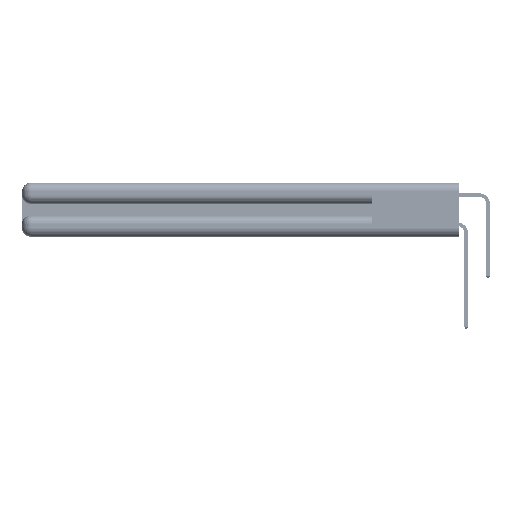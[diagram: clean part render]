
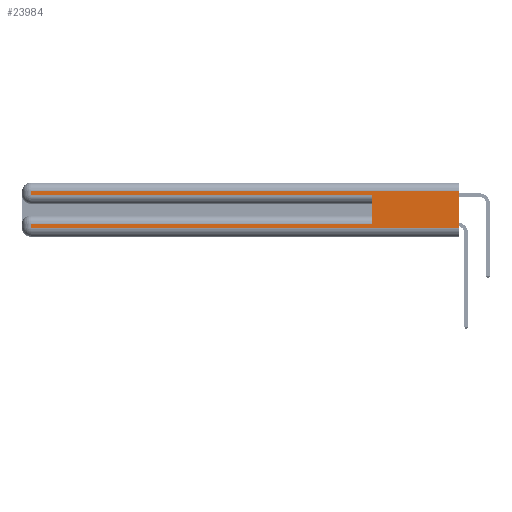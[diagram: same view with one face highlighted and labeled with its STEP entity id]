
A CAD part, left-side view. The second image highlights one B-rep face of the part: STEP entity #23984.
In plain terms, the highlighted planar face has unit normal (-1, 0, 0).
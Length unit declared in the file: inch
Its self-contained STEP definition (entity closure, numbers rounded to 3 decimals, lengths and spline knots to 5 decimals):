
#96 = FACE_OUTER_BOUND ( 'NONE', #7727, .T. ) ;
#660 = EDGE_CURVE ( 'NONE', #20867, #53211, #20556, .T. ) ;
#1240 = EDGE_CURVE ( 'NONE', #20867, #17692, #34169, .T. ) ;
#1460 = CARTESIAN_POINT ( 'NONE',  ( 0., 0., 0.06 ) ) ;
#1725 = LINE ( 'NONE', #55811, #45574 ) ;
#2793 = CARTESIAN_POINT ( 'NONE',  ( 0., 2.94, 0.37 ) ) ;
#4167 = VECTOR ( 'NONE', #28783, 39.37008 ) ;
#4797 = CARTESIAN_POINT ( 'NONE',  ( 0., 0., 0.31 ) ) ;
#5578 = CARTESIAN_POINT ( 'NONE',  ( 0., 0., 0.06 ) ) ;
#5601 = ORIENTED_EDGE ( 'NONE', *, *, #31787, .T. ) ;
#6433 = VECTOR ( 'NONE', #7778, 39.37008 ) ;
#7390 = CARTESIAN_POINT ( 'NONE',  ( 0., 0., 0.285 ) ) ;
#7727 = EDGE_LOOP ( 'NONE', ( #41674, #23294, #35686, #5601, #39688, #41686, #26981, #34441 ) ) ;
#7778 = DIRECTION ( 'NONE',  ( 0., -1., 0. ) ) ;
#8100 = DIRECTION ( 'NONE',  ( 1., 0., 0. ) ) ;
#8307 = LINE ( 'NONE', #28275, #26051 ) ;
#10941 = VECTOR ( 'NONE', #50600, 39.37008 ) ;
#12509 = VECTOR ( 'NONE', #22643, 39.37008 ) ;
#12558 = VERTEX_POINT ( 'NONE', #35543 ) ;
#12775 = VERTEX_POINT ( 'NONE', #15792 ) ;
#14449 = CARTESIAN_POINT ( 'NONE',  ( 0., 0., 0.085 ) ) ;
#15102 = VERTEX_POINT ( 'NONE', #45739 ) ;
#15792 = CARTESIAN_POINT ( 'NONE',  ( 0., 2.94, 0.285 ) ) ;
#17211 = VECTOR ( 'NONE', #40591, 39.37008 ) ;
#17470 = CARTESIAN_POINT ( 'NONE',  ( 0., 2.94, 0.31 ) ) ;
#17692 = VERTEX_POINT ( 'NONE', #1460 ) ;
#19238 = EDGE_CURVE ( 'NONE', #26409, #15102, #8307, .T. ) ;
#20556 = LINE ( 'NONE', #54392, #42480 ) ;
#20867 = VERTEX_POINT ( 'NONE', #4797 ) ;
#22643 = DIRECTION ( 'NONE',  ( 0., 1., 0. ) ) ;
#22738 = LINE ( 'NONE', #14449, #12509 ) ;
#23294 = ORIENTED_EDGE ( 'NONE', *, *, #660, .T. ) ;
#23572 = EDGE_CURVE ( 'NONE', #12558, #26409, #22738, .T. ) ;
#23984 = ADVANCED_FACE ( 'NONE', ( #96 ), #25264, .F. ) ;
#25075 = EDGE_CURVE ( 'NONE', #53211, #12775, #39094, .T. ) ;
#25264 = PLANE ( 'NONE',  #39997 ) ;
#26051 = VECTOR ( 'NONE', #43010, 39.37008 ) ;
#26409 = VERTEX_POINT ( 'NONE', #36772 ) ;
#26981 = ORIENTED_EDGE ( 'NONE', *, *, #19238, .T. ) ;
#28035 = EDGE_CURVE ( 'NONE', #12558, #34216, #1725, .T. ) ;
#28117 = DIRECTION ( 'NONE',  ( 0., 1., 0. ) ) ;
#28275 = CARTESIAN_POINT ( 'NONE',  ( 0., 2.94, 0.37 ) ) ;
#28783 = DIRECTION ( 'NONE',  ( 0., 0., -1. ) ) ;
#31787 = EDGE_CURVE ( 'NONE', #12775, #34216, #51623, .T. ) ;
#34169 = LINE ( 'NONE', #50782, #10941 ) ;
#34216 = VERTEX_POINT ( 'NONE', #39833 ) ;
#34277 = CARTESIAN_POINT ( 'NONE',  ( 0., 0., 0.37 ) ) ;
#34441 = ORIENTED_EDGE ( 'NONE', *, *, #53332, .T. ) ;
#35543 = CARTESIAN_POINT ( 'NONE',  ( 0., 0.6, 0.085 ) ) ;
#35686 = ORIENTED_EDGE ( 'NONE', *, *, #25075, .T. ) ;
#36772 = CARTESIAN_POINT ( 'NONE',  ( 0., 2.94, 0.085 ) ) ;
#38939 = DIRECTION ( 'NONE',  ( 0., 0., 1. ) ) ;
#39094 = LINE ( 'NONE', #2793, #4167 ) ;
#39688 = ORIENTED_EDGE ( 'NONE', *, *, #28035, .F. ) ;
#39833 = CARTESIAN_POINT ( 'NONE',  ( 0., 0.6, 0.285 ) ) ;
#39997 = AXIS2_PLACEMENT_3D ( 'NONE', #34277, #8100, #55955 ) ;
#40591 = DIRECTION ( 'NONE',  ( 0., -1., 0. ) ) ;
#41674 = ORIENTED_EDGE ( 'NONE', *, *, #1240, .F. ) ;
#41686 = ORIENTED_EDGE ( 'NONE', *, *, #23572, .T. ) ;
#42480 = VECTOR ( 'NONE', #28117, 39.37008 ) ;
#43010 = DIRECTION ( 'NONE',  ( 0., 0., -1. ) ) ;
#45279 = LINE ( 'NONE', #5578, #17211 ) ;
#45574 = VECTOR ( 'NONE', #38939, 39.37008 ) ;
#45739 = CARTESIAN_POINT ( 'NONE',  ( 0., 2.94, 0.06 ) ) ;
#50600 = DIRECTION ( 'NONE',  ( 0., 0., -1. ) ) ;
#50782 = CARTESIAN_POINT ( 'NONE',  ( 0., 0., 0.37 ) ) ;
#51623 = LINE ( 'NONE', #7390, #6433 ) ;
#53211 = VERTEX_POINT ( 'NONE', #17470 ) ;
#53332 = EDGE_CURVE ( 'NONE', #15102, #17692, #45279, .T. ) ;
#54392 = CARTESIAN_POINT ( 'NONE',  ( 0., 0., 0.31 ) ) ;
#55811 = CARTESIAN_POINT ( 'NONE',  ( 0., 0.6, 0.145 ) ) ;
#55955 = DIRECTION ( 'NONE',  ( 0., 0., -1. ) ) ;
